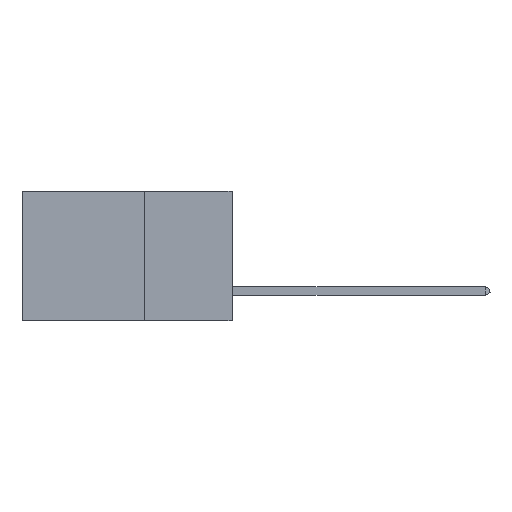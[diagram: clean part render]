
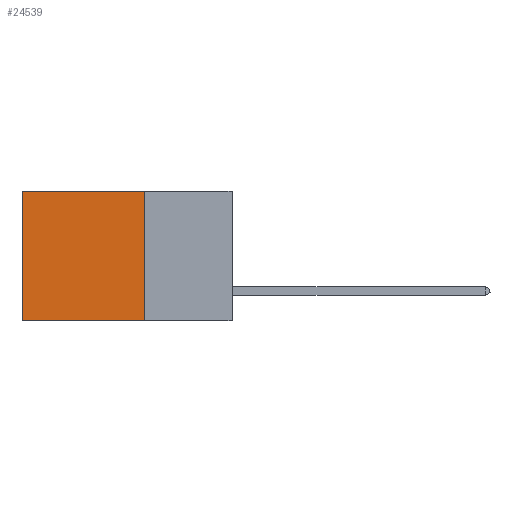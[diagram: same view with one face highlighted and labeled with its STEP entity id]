
A CAD part, left-side view. The second image highlights one B-rep face of the part: STEP entity #24539.
In plain terms, the highlighted planar face has unit normal (-1, 0, 0).
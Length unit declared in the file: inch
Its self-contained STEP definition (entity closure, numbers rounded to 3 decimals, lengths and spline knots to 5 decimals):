
#472 = VECTOR ( 'NONE', #1454, 39.37008 ) ;
#587 = VECTOR ( 'NONE', #19558, 39.37008 ) ;
#1454 = DIRECTION ( 'NONE',  ( 0., 1., 0. ) ) ;
#2642 = LINE ( 'NONE', #27439, #7064 ) ;
#6274 = VERTEX_POINT ( 'NONE', #25454 ) ;
#6981 = EDGE_CURVE ( 'NONE', #6274, #21232, #35637, .T. ) ;
#7064 = VECTOR ( 'NONE', #8032, 39.37008 ) ;
#7941 = CARTESIAN_POINT ( 'NONE',  ( 0.2875, 0.6, 0. ) ) ;
#7968 = AXIS2_PLACEMENT_3D ( 'NONE', #13768, #29130, #34809 ) ;
#8032 = DIRECTION ( 'NONE',  ( 0., 0., -1. ) ) ;
#9051 = EDGE_CURVE ( 'NONE', #25783, #21232, #11199, .T. ) ;
#11199 = LINE ( 'NONE', #28543, #587 ) ;
#13768 = CARTESIAN_POINT ( 'NONE',  ( 0.2875, 0.25, 0. ) ) ;
#13884 = PLANE ( 'NONE',  #7968 ) ;
#14348 = ORIENTED_EDGE ( 'NONE', *, *, #9051, .F. ) ;
#15560 = LINE ( 'NONE', #18456, #472 ) ;
#18456 = CARTESIAN_POINT ( 'NONE',  ( 0.2875, 0.25, 0. ) ) ;
#19558 = DIRECTION ( 'NONE',  ( 0., 1., 0. ) ) ;
#21232 = VERTEX_POINT ( 'NONE', #33443 ) ;
#21846 = VERTEX_POINT ( 'NONE', #29555 ) ;
#24539 = ADVANCED_FACE ( 'NONE', ( #25862 ), #13884, .F. ) ;
#25235 = ORIENTED_EDGE ( 'NONE', *, *, #28157, .F. ) ;
#25454 = CARTESIAN_POINT ( 'NONE',  ( 0.2875, 0.6, 0. ) ) ;
#25783 = VERTEX_POINT ( 'NONE', #33318 ) ;
#25862 = FACE_OUTER_BOUND ( 'NONE', #36210, .T. ) ;
#26587 = ORIENTED_EDGE ( 'NONE', *, *, #35369, .T. ) ;
#27439 = CARTESIAN_POINT ( 'NONE',  ( 0.2875, 0.25, 0. ) ) ;
#28157 = EDGE_CURVE ( 'NONE', #21846, #25783, #2642, .T. ) ;
#28543 = CARTESIAN_POINT ( 'NONE',  ( 0.2875, 0.25, -0.37 ) ) ;
#29130 = DIRECTION ( 'NONE',  ( 1., 0., 0. ) ) ;
#29555 = CARTESIAN_POINT ( 'NONE',  ( 0.2875, 0.25, 0. ) ) ;
#31250 = VECTOR ( 'NONE', #35716, 39.37008 ) ;
#33318 = CARTESIAN_POINT ( 'NONE',  ( 0.2875, 0.25, -0.37 ) ) ;
#33443 = CARTESIAN_POINT ( 'NONE',  ( 0.2875, 0.6, -0.37 ) ) ;
#34456 = ORIENTED_EDGE ( 'NONE', *, *, #6981, .T. ) ;
#34809 = DIRECTION ( 'NONE',  ( 0., 0., -1. ) ) ;
#35369 = EDGE_CURVE ( 'NONE', #21846, #6274, #15560, .T. ) ;
#35637 = LINE ( 'NONE', #7941, #31250 ) ;
#35716 = DIRECTION ( 'NONE',  ( 0., 0., -1. ) ) ;
#36210 = EDGE_LOOP ( 'NONE', ( #34456, #14348, #25235, #26587 ) ) ;
